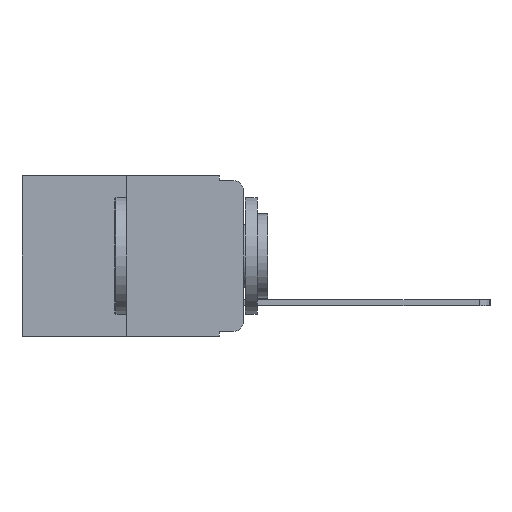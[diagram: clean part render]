
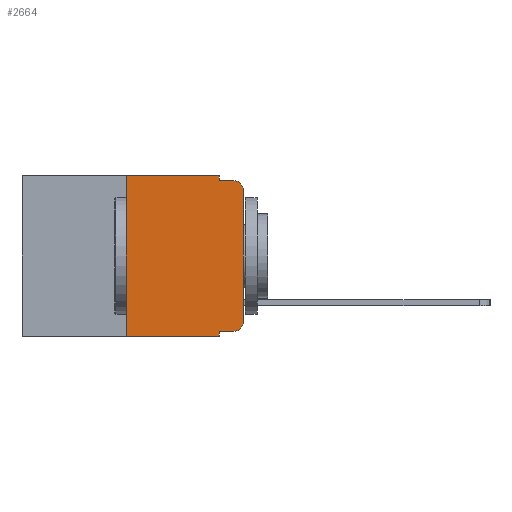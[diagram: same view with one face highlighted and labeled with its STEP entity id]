
A CAD part, left-side view. The second image highlights one B-rep face of the part: STEP entity #2664.
In plain terms, the highlighted planar face has unit normal (-1, 0, 0).
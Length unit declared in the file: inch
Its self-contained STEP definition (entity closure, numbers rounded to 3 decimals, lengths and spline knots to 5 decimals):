
#210 = VECTOR ( 'NONE', #15544, 39.37008 ) ;
#306 = VECTOR ( 'NONE', #2269, 39.37008 ) ;
#400 = EDGE_LOOP ( 'NONE', ( #10296, #13445, #3889, #16161, #6878, #14930, #12535, #11240, #9537, #14543 ) ) ;
#703 = CARTESIAN_POINT ( 'NONE',  ( 0., 0.051, -0.01 ) ) ;
#708 = LINE ( 'NONE', #887, #210 ) ;
#887 = CARTESIAN_POINT ( 'NONE',  ( 0., 0.473, -0.343 ) ) ;
#1072 = CARTESIAN_POINT ( 'NONE',  ( 0., 0.02, -0.333 ) ) ;
#1399 = DIRECTION ( 'NONE',  ( 0., 0., 1. ) ) ;
#1590 = EDGE_CURVE ( 'NONE', #10968, #7532, #6921, .T. ) ;
#2269 = DIRECTION ( 'NONE',  ( 0., -1., 0. ) ) ;
#2664 = ADVANCED_FACE ( 'NONE', ( #17513 ), #15892, .F. ) ;
#2774 = CARTESIAN_POINT ( 'NONE',  ( 0., 0.02, -0.313 ) ) ;
#3173 = EDGE_CURVE ( 'NONE', #3404, #10753, #708, .T. ) ;
#3404 = VERTEX_POINT ( 'NONE', #4685 ) ;
#3889 = ORIENTED_EDGE ( 'NONE', *, *, #6237, .F. ) ;
#3973 = CARTESIAN_POINT ( 'NONE',  ( 0., 0.25, 0. ) ) ;
#3984 = DIRECTION ( 'NONE',  ( 0., 0., 1. ) ) ;
#4021 = LINE ( 'NONE', #703, #306 ) ;
#4358 = DIRECTION ( 'NONE',  ( 0., 0., -1. ) ) ;
#4685 = CARTESIAN_POINT ( 'NONE',  ( 0., 0.25, -0.343 ) ) ;
#5626 = VERTEX_POINT ( 'NONE', #3973 ) ;
#5802 = EDGE_CURVE ( 'NONE', #8013, #7186, #8130, .T. ) ;
#5940 = CARTESIAN_POINT ( 'NONE',  ( 0., 0.473, 0. ) ) ;
#6194 = LINE ( 'NONE', #13045, #14020 ) ;
#6237 = EDGE_CURVE ( 'NONE', #9117, #7532, #4021, .T. ) ;
#6261 = DIRECTION ( 'NONE',  ( 0., 0., -1. ) ) ;
#6297 = DIRECTION ( 'NONE',  ( 0., 0., -1. ) ) ;
#6418 = LINE ( 'NONE', #18615, #13753 ) ;
#6878 = ORIENTED_EDGE ( 'NONE', *, *, #12294, .F. ) ;
#6921 = CIRCLE ( 'NONE', #16721, 0.02 ) ;
#7186 = VERTEX_POINT ( 'NONE', #12317 ) ;
#7523 = AXIS2_PLACEMENT_3D ( 'NONE', #18879, #19184, #17132 ) ;
#7532 = VERTEX_POINT ( 'NONE', #8906 ) ;
#7625 = EDGE_CURVE ( 'NONE', #12006, #9117, #13779, .T. ) ;
#8013 = VERTEX_POINT ( 'NONE', #1072 ) ;
#8130 = CIRCLE ( 'NONE', #12956, 0.02 ) ;
#8906 = CARTESIAN_POINT ( 'NONE',  ( 0., 0.02, -0.01 ) ) ;
#9117 = VERTEX_POINT ( 'NONE', #11029 ) ;
#9505 = LINE ( 'NONE', #13052, #16239 ) ;
#9537 = ORIENTED_EDGE ( 'NONE', *, *, #12768, .T. ) ;
#9643 = CARTESIAN_POINT ( 'NONE',  ( 0., 0., -0.03 ) ) ;
#10206 = VECTOR ( 'NONE', #18950, 39.37008 ) ;
#10296 = ORIENTED_EDGE ( 'NONE', *, *, #18344, .T. ) ;
#10389 = CARTESIAN_POINT ( 'NONE',  ( 0., 0.02, -0.03 ) ) ;
#10753 = VERTEX_POINT ( 'NONE', #17613 ) ;
#10968 = VERTEX_POINT ( 'NONE', #9643 ) ;
#11029 = CARTESIAN_POINT ( 'NONE',  ( 0., 0.051, -0.01 ) ) ;
#11240 = ORIENTED_EDGE ( 'NONE', *, *, #17187, .F. ) ;
#11696 = EDGE_CURVE ( 'NONE', #3404, #5626, #16720, .T. ) ;
#12006 = VERTEX_POINT ( 'NONE', #12624 ) ;
#12294 = EDGE_CURVE ( 'NONE', #5626, #12006, #14039, .T. ) ;
#12317 = CARTESIAN_POINT ( 'NONE',  ( 0., 0., -0.313 ) ) ;
#12535 = ORIENTED_EDGE ( 'NONE', *, *, #3173, .T. ) ;
#12624 = CARTESIAN_POINT ( 'NONE',  ( 0., 0.051, 0. ) ) ;
#12768 = EDGE_CURVE ( 'NONE', #13770, #8013, #6194, .T. ) ;
#12936 = VECTOR ( 'NONE', #1399, 39.37008 ) ;
#12956 = AXIS2_PLACEMENT_3D ( 'NONE', #2774, #13298, #4358 ) ;
#13045 = CARTESIAN_POINT ( 'NONE',  ( 0., 0.051, -0.333 ) ) ;
#13052 = CARTESIAN_POINT ( 'NONE',  ( 0., 0.051, 0. ) ) ;
#13298 = DIRECTION ( 'NONE',  ( -1., 0., 0. ) ) ;
#13445 = ORIENTED_EDGE ( 'NONE', *, *, #1590, .T. ) ;
#13449 = CARTESIAN_POINT ( 'NONE',  ( 0., 0.25, 0. ) ) ;
#13753 = VECTOR ( 'NONE', #3984, 39.37008 ) ;
#13770 = VERTEX_POINT ( 'NONE', #15543 ) ;
#13779 = LINE ( 'NONE', #15021, #17105 ) ;
#14020 = VECTOR ( 'NONE', #14498, 39.37008 ) ;
#14039 = LINE ( 'NONE', #5940, #10206 ) ;
#14498 = DIRECTION ( 'NONE',  ( 0., -1., 0. ) ) ;
#14543 = ORIENTED_EDGE ( 'NONE', *, *, #5802, .T. ) ;
#14930 = ORIENTED_EDGE ( 'NONE', *, *, #11696, .F. ) ;
#15021 = CARTESIAN_POINT ( 'NONE',  ( 0., 0.051, 0. ) ) ;
#15543 = CARTESIAN_POINT ( 'NONE',  ( 0., 0.051, -0.333 ) ) ;
#15544 = DIRECTION ( 'NONE',  ( 0., -1., 0. ) ) ;
#15840 = DIRECTION ( 'NONE',  ( 0., 0., -1. ) ) ;
#15892 = PLANE ( 'NONE',  #7523 ) ;
#16161 = ORIENTED_EDGE ( 'NONE', *, *, #7625, .F. ) ;
#16239 = VECTOR ( 'NONE', #15840, 39.37008 ) ;
#16720 = LINE ( 'NONE', #13449, #12936 ) ;
#16721 = AXIS2_PLACEMENT_3D ( 'NONE', #10389, #17503, #6297 ) ;
#17105 = VECTOR ( 'NONE', #6261, 39.37008 ) ;
#17132 = DIRECTION ( 'NONE',  ( 0., 0., -1. ) ) ;
#17187 = EDGE_CURVE ( 'NONE', #13770, #10753, #9505, .T. ) ;
#17503 = DIRECTION ( 'NONE',  ( -1., 0., 0. ) ) ;
#17513 = FACE_OUTER_BOUND ( 'NONE', #400, .T. ) ;
#17613 = CARTESIAN_POINT ( 'NONE',  ( 0., 0.051, -0.343 ) ) ;
#18344 = EDGE_CURVE ( 'NONE', #7186, #10968, #6418, .T. ) ;
#18615 = CARTESIAN_POINT ( 'NONE',  ( 0., 0., 0. ) ) ;
#18879 = CARTESIAN_POINT ( 'NONE',  ( 0., 0.473, 0. ) ) ;
#18950 = DIRECTION ( 'NONE',  ( 0., -1., 0. ) ) ;
#19184 = DIRECTION ( 'NONE',  ( 1., 0., 0. ) ) ;
